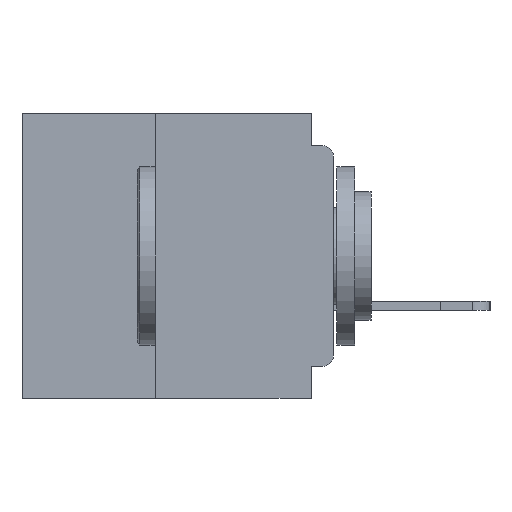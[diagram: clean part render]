
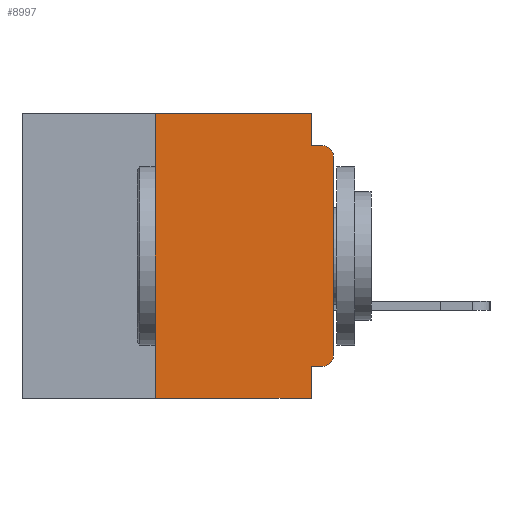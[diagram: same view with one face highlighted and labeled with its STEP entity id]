
A CAD part, left-side view. The second image highlights one B-rep face of the part: STEP entity #8997.
In plain terms, the highlighted planar face has unit normal (-1, 0, 0).
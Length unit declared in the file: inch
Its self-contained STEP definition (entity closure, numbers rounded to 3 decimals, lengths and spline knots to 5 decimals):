
#221 = DIRECTION ( 'NONE',  ( 0., 0., -1. ) ) ;
#1700 = ORIENTED_EDGE ( 'NONE', *, *, #11777, .F. ) ;
#1994 = DIRECTION ( 'NONE',  ( -1., 0., 0. ) ) ;
#2669 = ORIENTED_EDGE ( 'NONE', *, *, #26945, .F. ) ;
#3069 = ORIENTED_EDGE ( 'NONE', *, *, #32240, .T. ) ;
#3822 = CARTESIAN_POINT ( 'NONE',  ( 0., 0.031, -0.045 ) ) ;
#4577 = LINE ( 'NONE', #27836, #27715 ) ;
#5532 = DIRECTION ( 'NONE',  ( 0., 0., 1. ) ) ;
#6254 = CARTESIAN_POINT ( 'NONE',  ( 0., 0.031, 0. ) ) ;
#7689 = EDGE_CURVE ( 'NONE', #21395, #37884, #15024, .T. ) ;
#7969 = EDGE_CURVE ( 'NONE', #7990, #9818, #4577, .T. ) ;
#7990 = VERTEX_POINT ( 'NONE', #3822 ) ;
#8020 = CARTESIAN_POINT ( 'NONE',  ( 0., 0.015, -0.355 ) ) ;
#8028 = DIRECTION ( 'NONE',  ( -1., 0., 0. ) ) ;
#8174 = CIRCLE ( 'NONE', #21052, 0.015 ) ;
#8360 = PLANE ( 'NONE',  #35250 ) ;
#8499 = EDGE_LOOP ( 'NONE', ( #3069, #20140, #13037, #1700, #19695, #12581, #18294, #10224, #2669, #29547 ) ) ;
#8969 = VECTOR ( 'NONE', #29651, 39.37008 ) ;
#8997 = ADVANCED_FACE ( 'NONE', ( #18330 ), #8360, .F. ) ;
#9041 = VERTEX_POINT ( 'NONE', #23680 ) ;
#9736 = EDGE_CURVE ( 'NONE', #21395, #9041, #34737, .T. ) ;
#9783 = DIRECTION ( 'NONE',  ( 0., -1., 0. ) ) ;
#9818 = VERTEX_POINT ( 'NONE', #36130 ) ;
#10056 = CARTESIAN_POINT ( 'NONE',  ( 0., 0.25, -0.4 ) ) ;
#10147 = DIRECTION ( 'NONE',  ( 0., 0., -1. ) ) ;
#10224 = ORIENTED_EDGE ( 'NONE', *, *, #38743, .F. ) ;
#10999 = DIRECTION ( 'NONE',  ( 0., -1., 0. ) ) ;
#11453 = VECTOR ( 'NONE', #221, 39.37008 ) ;
#11777 = EDGE_CURVE ( 'NONE', #30191, #7990, #34561, .T. ) ;
#11804 = CARTESIAN_POINT ( 'NONE',  ( 0., 0.031, -0.4 ) ) ;
#12581 = ORIENTED_EDGE ( 'NONE', *, *, #9736, .F. ) ;
#12810 = EDGE_CURVE ( 'NONE', #28150, #21174, #31614, .T. ) ;
#12940 = EDGE_CURVE ( 'NONE', #9041, #30191, #25964, .T. ) ;
#13037 = ORIENTED_EDGE ( 'NONE', *, *, #7969, .F. ) ;
#13377 = AXIS2_PLACEMENT_3D ( 'NONE', #26130, #8028, #29141 ) ;
#13841 = VECTOR ( 'NONE', #23184, 39.37008 ) ;
#14033 = CARTESIAN_POINT ( 'NONE',  ( 0., 0.437, -0.4 ) ) ;
#14427 = VECTOR ( 'NONE', #10147, 39.37008 ) ;
#14457 = CARTESIAN_POINT ( 'NONE',  ( 0., 0.437, 0. ) ) ;
#15024 = LINE ( 'NONE', #14033, #23972 ) ;
#15739 = LINE ( 'NONE', #34029, #30778 ) ;
#16414 = CARTESIAN_POINT ( 'NONE',  ( 0., 0., -0.06 ) ) ;
#16854 = EDGE_CURVE ( 'NONE', #33814, #9818, #8174, .T. ) ;
#17443 = VERTEX_POINT ( 'NONE', #29479 ) ;
#17509 = DIRECTION ( 'NONE',  ( 0., 0., -1. ) ) ;
#17877 = CARTESIAN_POINT ( 'NONE',  ( 0., 0., -0.34 ) ) ;
#18294 = ORIENTED_EDGE ( 'NONE', *, *, #7689, .T. ) ;
#18330 = FACE_OUTER_BOUND ( 'NONE', #8499, .T. ) ;
#19695 = ORIENTED_EDGE ( 'NONE', *, *, #12940, .F. ) ;
#20113 = CARTESIAN_POINT ( 'NONE',  ( 0., 0.015, -0.06 ) ) ;
#20140 = ORIENTED_EDGE ( 'NONE', *, *, #16854, .T. ) ;
#20191 = CARTESIAN_POINT ( 'NONE',  ( 0., 0., 0. ) ) ;
#20618 = CARTESIAN_POINT ( 'NONE',  ( 0., 0.437, 0. ) ) ;
#21052 = AXIS2_PLACEMENT_3D ( 'NONE', #20113, #1994, #23094 ) ;
#21174 = VERTEX_POINT ( 'NONE', #17877 ) ;
#21395 = VERTEX_POINT ( 'NONE', #10056 ) ;
#21641 = CARTESIAN_POINT ( 'NONE',  ( 0., 0.031, 0. ) ) ;
#21858 = LINE ( 'NONE', #20191, #13841 ) ;
#22424 = LINE ( 'NONE', #34132, #14427 ) ;
#23094 = DIRECTION ( 'NONE',  ( 0., 0., -1. ) ) ;
#23184 = DIRECTION ( 'NONE',  ( 0., 0., 1. ) ) ;
#23680 = CARTESIAN_POINT ( 'NONE',  ( 0., 0.25, 0. ) ) ;
#23972 = VECTOR ( 'NONE', #10999, 39.37008 ) ;
#25964 = LINE ( 'NONE', #20618, #8969 ) ;
#26130 = CARTESIAN_POINT ( 'NONE',  ( 0., 0.015, -0.34 ) ) ;
#26945 = EDGE_CURVE ( 'NONE', #28150, #17443, #15739, .T. ) ;
#27715 = VECTOR ( 'NONE', #9783, 39.37008 ) ;
#27836 = CARTESIAN_POINT ( 'NONE',  ( 0., 0., -0.045 ) ) ;
#28090 = DIRECTION ( 'NONE',  ( 0., 1., 0. ) ) ;
#28150 = VERTEX_POINT ( 'NONE', #8020 ) ;
#29141 = DIRECTION ( 'NONE',  ( 0., 0., -1. ) ) ;
#29479 = CARTESIAN_POINT ( 'NONE',  ( 0., 0.031, -0.355 ) ) ;
#29547 = ORIENTED_EDGE ( 'NONE', *, *, #12810, .T. ) ;
#29651 = DIRECTION ( 'NONE',  ( 0., -1., 0. ) ) ;
#30191 = VERTEX_POINT ( 'NONE', #21641 ) ;
#30778 = VECTOR ( 'NONE', #28090, 39.37008 ) ;
#31614 = CIRCLE ( 'NONE', #13377, 0.015 ) ;
#31873 = VECTOR ( 'NONE', #5532, 39.37008 ) ;
#32240 = EDGE_CURVE ( 'NONE', #21174, #33814, #21858, .T. ) ;
#33814 = VERTEX_POINT ( 'NONE', #16414 ) ;
#34029 = CARTESIAN_POINT ( 'NONE',  ( 0., 0., -0.355 ) ) ;
#34132 = CARTESIAN_POINT ( 'NONE',  ( 0., 0.031, -0.4 ) ) ;
#34561 = LINE ( 'NONE', #6254, #11453 ) ;
#34737 = LINE ( 'NONE', #38747, #31873 ) ;
#35250 = AXIS2_PLACEMENT_3D ( 'NONE', #14457, #35545, #17509 ) ;
#35545 = DIRECTION ( 'NONE',  ( 1., 0., 0. ) ) ;
#36130 = CARTESIAN_POINT ( 'NONE',  ( 0., 0.015, -0.045 ) ) ;
#37884 = VERTEX_POINT ( 'NONE', #11804 ) ;
#38743 = EDGE_CURVE ( 'NONE', #17443, #37884, #22424, .T. ) ;
#38747 = CARTESIAN_POINT ( 'NONE',  ( 0., 0.25, -0.4 ) ) ;
